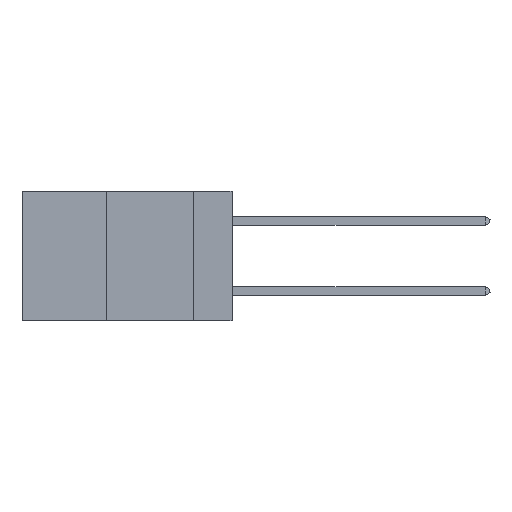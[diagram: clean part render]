
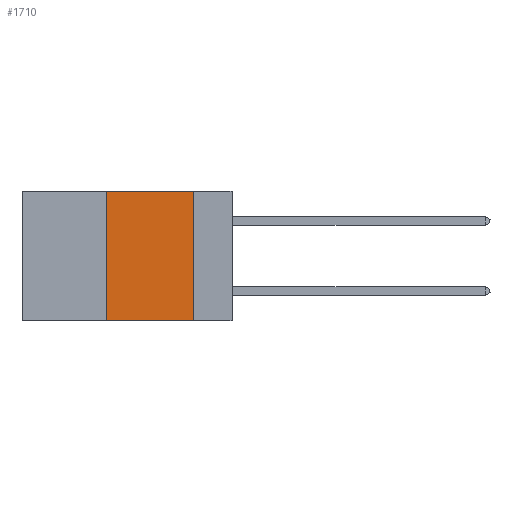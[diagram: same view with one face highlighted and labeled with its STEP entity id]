
A CAD part, left-side view. The second image highlights one B-rep face of the part: STEP entity #1710.
In plain terms, the highlighted planar face has unit normal (-1, 0, 0).
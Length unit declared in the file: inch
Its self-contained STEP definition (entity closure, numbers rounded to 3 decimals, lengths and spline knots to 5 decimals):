
#610 = CARTESIAN_POINT ( 'NONE',  ( 0., 0.36, -0.37 ) ) ;
#1710 = ADVANCED_FACE ( 'NONE', ( #6354 ), #23159, .F. ) ;
#2185 = CARTESIAN_POINT ( 'NONE',  ( 0., 0.11, -0.37 ) ) ;
#4366 = DIRECTION ( 'NONE',  ( 0., 0., -1. ) ) ;
#6354 = FACE_OUTER_BOUND ( 'NONE', #14207, .T. ) ;
#6530 = EDGE_CURVE ( 'NONE', #36680, #18332, #7677, .T. ) ;
#7677 = LINE ( 'NONE', #42723, #24360 ) ;
#9212 = EDGE_CURVE ( 'NONE', #18332, #45333, #33791, .T. ) ;
#9880 = ORIENTED_EDGE ( 'NONE', *, *, #6530, .F. ) ;
#11137 = EDGE_CURVE ( 'NONE', #45333, #25102, #36583, .T. ) ;
#12499 = DIRECTION ( 'NONE',  ( 0., -1., 0. ) ) ;
#14207 = EDGE_LOOP ( 'NONE', ( #39878, #19718, #9880, #29435 ) ) ;
#14792 = VECTOR ( 'NONE', #12499, 39.37008 ) ;
#16188 = EDGE_CURVE ( 'NONE', #36680, #25102, #21720, .T. ) ;
#18129 = VECTOR ( 'NONE', #20684, 39.37008 ) ;
#18332 = VERTEX_POINT ( 'NONE', #35285 ) ;
#19718 = ORIENTED_EDGE ( 'NONE', *, *, #9212, .F. ) ;
#20684 = DIRECTION ( 'NONE',  ( 0., -1., 0. ) ) ;
#21720 = LINE ( 'NONE', #24499, #18129 ) ;
#22834 = CARTESIAN_POINT ( 'NONE',  ( 0., 0.6, 0. ) ) ;
#23159 = PLANE ( 'NONE',  #26463 ) ;
#24360 = VECTOR ( 'NONE', #31154, 39.37008 ) ;
#24499 = CARTESIAN_POINT ( 'NONE',  ( 0., 0.6, -0.37 ) ) ;
#25102 = VERTEX_POINT ( 'NONE', #2185 ) ;
#26463 = AXIS2_PLACEMENT_3D ( 'NONE', #22834, #27119, #4366 ) ;
#26476 = VECTOR ( 'NONE', #27777, 39.37008 ) ;
#27119 = DIRECTION ( 'NONE',  ( 1., 0., 0. ) ) ;
#27610 = CARTESIAN_POINT ( 'NONE',  ( 0., 0.6, 0. ) ) ;
#27777 = DIRECTION ( 'NONE',  ( 0., 0., -1. ) ) ;
#29435 = ORIENTED_EDGE ( 'NONE', *, *, #16188, .T. ) ;
#31154 = DIRECTION ( 'NONE',  ( 0., 0., 1. ) ) ;
#32934 = CARTESIAN_POINT ( 'NONE',  ( 0., 0.11, 0. ) ) ;
#33791 = LINE ( 'NONE', #27610, #14792 ) ;
#35285 = CARTESIAN_POINT ( 'NONE',  ( 0., 0.36, 0. ) ) ;
#36583 = LINE ( 'NONE', #38561, #26476 ) ;
#36680 = VERTEX_POINT ( 'NONE', #610 ) ;
#38561 = CARTESIAN_POINT ( 'NONE',  ( 0., 0.11, 0. ) ) ;
#39878 = ORIENTED_EDGE ( 'NONE', *, *, #11137, .F. ) ;
#42723 = CARTESIAN_POINT ( 'NONE',  ( 0., 0.36, 0. ) ) ;
#45333 = VERTEX_POINT ( 'NONE', #32934 ) ;
